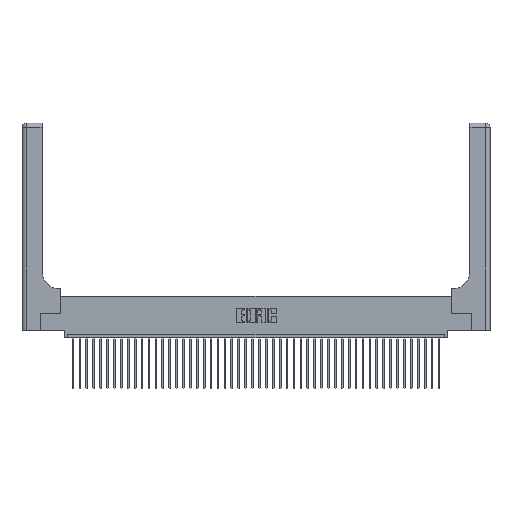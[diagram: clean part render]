
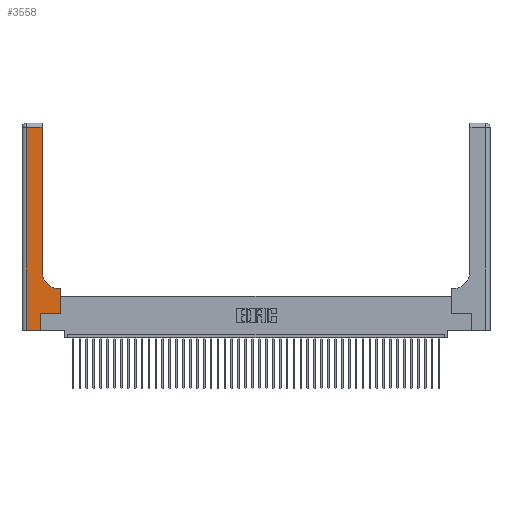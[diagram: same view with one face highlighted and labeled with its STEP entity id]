
A CAD part, top view. The second image highlights one B-rep face of the part: STEP entity #3558.
In plain terms, the highlighted planar face has unit normal (0, 0, 1).
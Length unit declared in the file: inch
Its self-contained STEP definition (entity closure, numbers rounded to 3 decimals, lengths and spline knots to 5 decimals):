
#1880 = AXIS2_PLACEMENT_3D ( 'NONE', #12109, #43071, #15380 ) ;
#3465 = VERTEX_POINT ( 'NONE', #26762 ) ;
#3558 = ADVANCED_FACE ( 'NONE', ( #33852 ), #30501, .F. ) ;
#3718 = DIRECTION ( 'NONE',  ( 1., 0., 0. ) ) ;
#5153 = CARTESIAN_POINT ( 'NONE',  ( 0.269, 0.25, 0.37 ) ) ;
#5417 = AXIS2_PLACEMENT_3D ( 'NONE', #41950, #28456, #35324 ) ;
#6699 = VERTEX_POINT ( 'NONE', #5153 ) ;
#7189 = ORIENTED_EDGE ( 'NONE', *, *, #12194, .T. ) ;
#7852 = CARTESIAN_POINT ( 'NONE',  ( 0.269, 0., 0.37 ) ) ;
#8423 = CARTESIAN_POINT ( 'NONE',  ( 0.2915, 2.94, 0.37 ) ) ;
#8813 = VECTOR ( 'NONE', #3718, 39.37008 ) ;
#9564 = EDGE_CURVE ( 'NONE', #33306, #3465, #21805, .T. ) ;
#10370 = EDGE_CURVE ( 'NONE', #11314, #17730, #20155, .T. ) ;
#10617 = DIRECTION ( 'NONE',  ( -1., 0., 0. ) ) ;
#11314 = VERTEX_POINT ( 'NONE', #35383 ) ;
#11426 = CARTESIAN_POINT ( 'NONE',  ( 0.2915, 3., 0.37 ) ) ;
#12065 = DIRECTION ( 'NONE',  ( 0., 1., 0. ) ) ;
#12109 = CARTESIAN_POINT ( 'NONE',  ( 0.5415, 0.85, 0.37 ) ) ;
#12194 = EDGE_CURVE ( 'NONE', #3465, #11314, #30165, .T. ) ;
#13284 = LINE ( 'NONE', #30934, #18074 ) ;
#13288 = EDGE_CURVE ( 'NONE', #23410, #6699, #25251, .T. ) ;
#13714 = EDGE_CURVE ( 'NONE', #6699, #33306, #26330, .T. ) ;
#15380 = DIRECTION ( 'NONE',  ( 1., 0., 0. ) ) ;
#15694 = ORIENTED_EDGE ( 'NONE', *, *, #30792, .T. ) ;
#16577 = ORIENTED_EDGE ( 'NONE', *, *, #27729, .T. ) ;
#16710 = CARTESIAN_POINT ( 'NONE',  ( 0.06, 3., 0.37 ) ) ;
#17354 = CARTESIAN_POINT ( 'NONE',  ( 0.2915, 0.6, 0.37 ) ) ;
#17730 = VERTEX_POINT ( 'NONE', #23271 ) ;
#18074 = VECTOR ( 'NONE', #27625, 39.37008 ) ;
#18955 = CARTESIAN_POINT ( 'NONE',  ( 0.269, 0., 0.37 ) ) ;
#18961 = CARTESIAN_POINT ( 'NONE',  ( 0.5585, 0.25, 0.37 ) ) ;
#19641 = VERTEX_POINT ( 'NONE', #8423 ) ;
#20155 = CIRCLE ( 'NONE', #1880, 0.25 ) ;
#20631 = ORIENTED_EDGE ( 'NONE', *, *, #13288, .T. ) ;
#21633 = EDGE_LOOP ( 'NONE', ( #16577, #41215, #15694, #40909, #20631, #40165, #43434, #7189, #28489 ) ) ;
#21805 = LINE ( 'NONE', #18961, #42224 ) ;
#21889 = EDGE_CURVE ( 'NONE', #44150, #23410, #39935, .T. ) ;
#22225 = DIRECTION ( 'NONE',  ( 0., 1., 0. ) ) ;
#23267 = CARTESIAN_POINT ( 'NONE',  ( 0.06, 0., 0.37 ) ) ;
#23271 = CARTESIAN_POINT ( 'NONE',  ( 0.2915, 0.85, 0.37 ) ) ;
#23410 = VERTEX_POINT ( 'NONE', #7852 ) ;
#23646 = VECTOR ( 'NONE', #31980, 39.37008 ) ;
#23838 = CARTESIAN_POINT ( 'NONE',  ( 0.5585, 0.25, 0.37 ) ) ;
#25251 = LINE ( 'NONE', #18955, #28512 ) ;
#25975 = CARTESIAN_POINT ( 'NONE',  ( 0.06, 2.94, 0.37 ) ) ;
#26330 = LINE ( 'NONE', #42184, #23646 ) ;
#26528 = DIRECTION ( 'NONE',  ( 0., -1., 0. ) ) ;
#26762 = CARTESIAN_POINT ( 'NONE',  ( 0.5585, 0.6, 0.37 ) ) ;
#26812 = LINE ( 'NONE', #16710, #31068 ) ;
#27625 = DIRECTION ( 'NONE',  ( -1., 0., 0. ) ) ;
#27729 = EDGE_CURVE ( 'NONE', #17730, #19641, #37761, .T. ) ;
#28456 = DIRECTION ( 'NONE',  ( 0., 0., -1. ) ) ;
#28489 = ORIENTED_EDGE ( 'NONE', *, *, #10370, .T. ) ;
#28512 = VECTOR ( 'NONE', #28739, 39.37008 ) ;
#28556 = VECTOR ( 'NONE', #10617, 39.37008 ) ;
#28739 = DIRECTION ( 'NONE',  ( 0., 1., 0. ) ) ;
#29054 = CARTESIAN_POINT ( 'NONE',  ( 0., 0., 0.37 ) ) ;
#30165 = LINE ( 'NONE', #17354, #28556 ) ;
#30501 = PLANE ( 'NONE',  #5417 ) ;
#30792 = EDGE_CURVE ( 'NONE', #40597, #44150, #26812, .T. ) ;
#30934 = CARTESIAN_POINT ( 'NONE',  ( 0., 2.94, 0.37 ) ) ;
#31068 = VECTOR ( 'NONE', #26528, 39.37008 ) ;
#31605 = EDGE_CURVE ( 'NONE', #19641, #40597, #13284, .T. ) ;
#31980 = DIRECTION ( 'NONE',  ( 1., 0., 0. ) ) ;
#33306 = VERTEX_POINT ( 'NONE', #23838 ) ;
#33852 = FACE_OUTER_BOUND ( 'NONE', #21633, .T. ) ;
#34550 = VECTOR ( 'NONE', #22225, 39.37008 ) ;
#35324 = DIRECTION ( 'NONE',  ( -1., 0., 0. ) ) ;
#35383 = CARTESIAN_POINT ( 'NONE',  ( 0.5415, 0.6, 0.37 ) ) ;
#37761 = LINE ( 'NONE', #11426, #34550 ) ;
#39935 = LINE ( 'NONE', #29054, #8813 ) ;
#40165 = ORIENTED_EDGE ( 'NONE', *, *, #13714, .T. ) ;
#40597 = VERTEX_POINT ( 'NONE', #25975 ) ;
#40909 = ORIENTED_EDGE ( 'NONE', *, *, #21889, .T. ) ;
#41215 = ORIENTED_EDGE ( 'NONE', *, *, #31605, .T. ) ;
#41950 = CARTESIAN_POINT ( 'NONE',  ( 0., 3., 0.37 ) ) ;
#42184 = CARTESIAN_POINT ( 'NONE',  ( 0.269, 0.25, 0.37 ) ) ;
#42224 = VECTOR ( 'NONE', #12065, 39.37008 ) ;
#43071 = DIRECTION ( 'NONE',  ( 0., 0., -1. ) ) ;
#43434 = ORIENTED_EDGE ( 'NONE', *, *, #9564, .T. ) ;
#44150 = VERTEX_POINT ( 'NONE', #23267 ) ;
